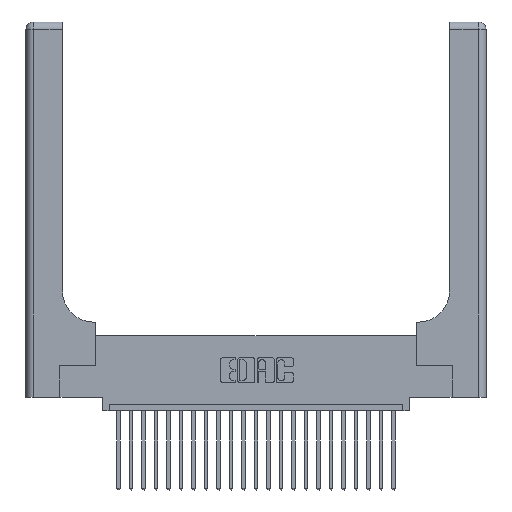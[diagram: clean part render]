
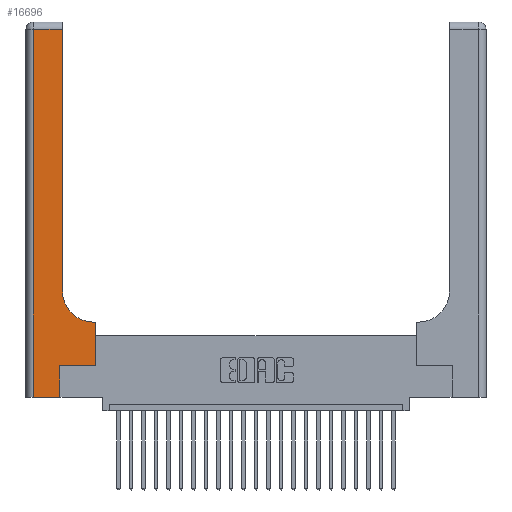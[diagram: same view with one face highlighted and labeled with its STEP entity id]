
A CAD part, top view. The second image highlights one B-rep face of the part: STEP entity #16696.
In plain terms, the highlighted planar face has unit normal (0, 0, 1).
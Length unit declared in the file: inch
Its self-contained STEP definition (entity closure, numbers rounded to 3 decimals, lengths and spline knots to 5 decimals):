
#193 = VERTEX_POINT ( 'NONE', #22268 ) ;
#1620 = EDGE_LOOP ( 'NONE', ( #17491, #6344, #5075, #14439, #20626, #10278, #6463, #1980, #6319 ) ) ;
#1635 = CARTESIAN_POINT ( 'NONE',  ( 0.269, 0.25, 0.37 ) ) ;
#1660 = DIRECTION ( 'NONE',  ( -1., 0., 0. ) ) ;
#1897 = EDGE_CURVE ( 'NONE', #22491, #18438, #9752, .T. ) ;
#1980 = ORIENTED_EDGE ( 'NONE', *, *, #22645, .T. ) ;
#1983 = DIRECTION ( 'NONE',  ( 0., -1., 0. ) ) ;
#2411 = EDGE_CURVE ( 'NONE', #193, #22757, #4228, .T. ) ;
#2632 = DIRECTION ( 'NONE',  ( 0., 0., -1. ) ) ;
#2926 = CARTESIAN_POINT ( 'NONE',  ( 0.2915, 2.94, 0.37 ) ) ;
#3533 = CARTESIAN_POINT ( 'NONE',  ( 0.2915, 0.6, 0.37 ) ) ;
#3672 = CARTESIAN_POINT ( 'NONE',  ( 0.5585, 0.25, 0.37 ) ) ;
#3804 = LINE ( 'NONE', #1635, #22979 ) ;
#4228 = CIRCLE ( 'NONE', #5865, 0.25 ) ;
#4425 = EDGE_CURVE ( 'NONE', #7505, #6067, #14826, .T. ) ;
#5075 = ORIENTED_EDGE ( 'NONE', *, *, #1897, .T. ) ;
#5770 = CARTESIAN_POINT ( 'NONE',  ( 0.2915, 0.85, 0.37 ) ) ;
#5865 = AXIS2_PLACEMENT_3D ( 'NONE', #20344, #2632, #12475 ) ;
#6000 = CARTESIAN_POINT ( 'NONE',  ( 0.06, 3., 0.37 ) ) ;
#6067 = VERTEX_POINT ( 'NONE', #21703 ) ;
#6319 = ORIENTED_EDGE ( 'NONE', *, *, #2411, .T. ) ;
#6344 = ORIENTED_EDGE ( 'NONE', *, *, #17716, .T. ) ;
#6349 = DIRECTION ( 'NONE',  ( -1., 0., 0. ) ) ;
#6434 = PLANE ( 'NONE',  #12597 ) ;
#6463 = ORIENTED_EDGE ( 'NONE', *, *, #4425, .T. ) ;
#6641 = DIRECTION ( 'NONE',  ( 1., 0., 0. ) ) ;
#7505 = VERTEX_POINT ( 'NONE', #3672 ) ;
#8026 = LINE ( 'NONE', #20329, #19037 ) ;
#8403 = VECTOR ( 'NONE', #24329, 39.37008 ) ;
#8538 = VERTEX_POINT ( 'NONE', #16051 ) ;
#8968 = CARTESIAN_POINT ( 'NONE',  ( 0.269, 0., 0.37 ) ) ;
#9147 = FACE_OUTER_BOUND ( 'NONE', #1620, .T. ) ;
#9752 = LINE ( 'NONE', #6000, #17649 ) ;
#10192 = CARTESIAN_POINT ( 'NONE',  ( 0.2915, 3., 0.37 ) ) ;
#10278 = ORIENTED_EDGE ( 'NONE', *, *, #23399, .T. ) ;
#10480 = DIRECTION ( 'NONE',  ( 0., 0., -1. ) ) ;
#10955 = VERTEX_POINT ( 'NONE', #2926 ) ;
#11566 = DIRECTION ( 'NONE',  ( 1., 0., 0. ) ) ;
#12047 = EDGE_CURVE ( 'NONE', #22757, #10955, #16681, .T. ) ;
#12127 = DIRECTION ( 'NONE',  ( 0., 1., 0. ) ) ;
#12367 = DIRECTION ( 'NONE',  ( -1., 0., 0. ) ) ;
#12475 = DIRECTION ( 'NONE',  ( 1., 0., 0. ) ) ;
#12597 = AXIS2_PLACEMENT_3D ( 'NONE', #16104, #10480, #6349 ) ;
#13053 = VERTEX_POINT ( 'NONE', #20228 ) ;
#13291 = EDGE_CURVE ( 'NONE', #8538, #13053, #16949, .T. ) ;
#14203 = VECTOR ( 'NONE', #12127, 39.37008 ) ;
#14439 = ORIENTED_EDGE ( 'NONE', *, *, #22087, .T. ) ;
#14476 = VECTOR ( 'NONE', #1660, 39.37008 ) ;
#14826 = LINE ( 'NONE', #16612, #21563 ) ;
#16051 = CARTESIAN_POINT ( 'NONE',  ( 0.269, 0., 0.37 ) ) ;
#16104 = CARTESIAN_POINT ( 'NONE',  ( 0., 3., 0.37 ) ) ;
#16351 = DIRECTION ( 'NONE',  ( 0., 1., 0. ) ) ;
#16612 = CARTESIAN_POINT ( 'NONE',  ( 0.5585, 0.25, 0.37 ) ) ;
#16681 = LINE ( 'NONE', #10192, #14203 ) ;
#16696 = ADVANCED_FACE ( 'NONE', ( #9147 ), #6434, .F. ) ;
#16949 = LINE ( 'NONE', #8968, #8403 ) ;
#17491 = ORIENTED_EDGE ( 'NONE', *, *, #12047, .T. ) ;
#17649 = VECTOR ( 'NONE', #1983, 39.37008 ) ;
#17716 = EDGE_CURVE ( 'NONE', #10955, #22491, #8026, .T. ) ;
#18438 = VERTEX_POINT ( 'NONE', #25003 ) ;
#19037 = VECTOR ( 'NONE', #12367, 39.37008 ) ;
#19697 = LINE ( 'NONE', #3533, #14476 ) ;
#20228 = CARTESIAN_POINT ( 'NONE',  ( 0.269, 0.25, 0.37 ) ) ;
#20329 = CARTESIAN_POINT ( 'NONE',  ( 0., 2.94, 0.37 ) ) ;
#20344 = CARTESIAN_POINT ( 'NONE',  ( 0.5415, 0.85, 0.37 ) ) ;
#20626 = ORIENTED_EDGE ( 'NONE', *, *, #13291, .T. ) ;
#21563 = VECTOR ( 'NONE', #16351, 39.37008 ) ;
#21703 = CARTESIAN_POINT ( 'NONE',  ( 0.5585, 0.6, 0.37 ) ) ;
#22087 = EDGE_CURVE ( 'NONE', #18438, #8538, #23032, .T. ) ;
#22268 = CARTESIAN_POINT ( 'NONE',  ( 0.5415, 0.6, 0.37 ) ) ;
#22491 = VERTEX_POINT ( 'NONE', #22677 ) ;
#22645 = EDGE_CURVE ( 'NONE', #6067, #193, #19697, .T. ) ;
#22677 = CARTESIAN_POINT ( 'NONE',  ( 0.06, 2.94, 0.37 ) ) ;
#22742 = VECTOR ( 'NONE', #6641, 39.37008 ) ;
#22757 = VERTEX_POINT ( 'NONE', #5770 ) ;
#22979 = VECTOR ( 'NONE', #11566, 39.37008 ) ;
#23032 = LINE ( 'NONE', #23922, #22742 ) ;
#23399 = EDGE_CURVE ( 'NONE', #13053, #7505, #3804, .T. ) ;
#23922 = CARTESIAN_POINT ( 'NONE',  ( 0., 0., 0.37 ) ) ;
#24329 = DIRECTION ( 'NONE',  ( 0., 1., 0. ) ) ;
#25003 = CARTESIAN_POINT ( 'NONE',  ( 0.06, 0., 0.37 ) ) ;
